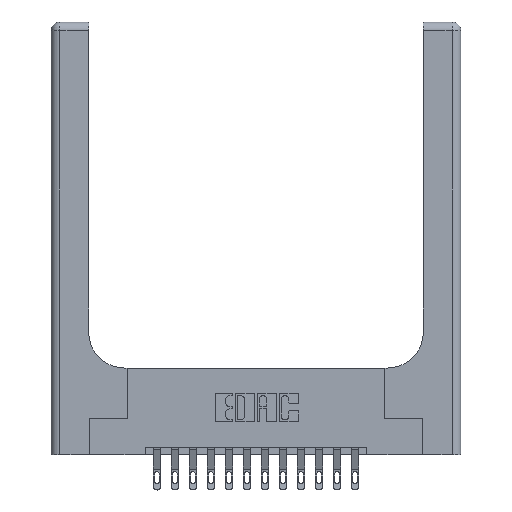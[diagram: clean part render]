
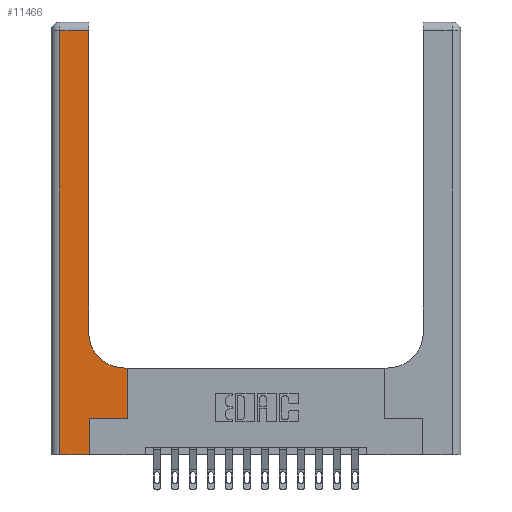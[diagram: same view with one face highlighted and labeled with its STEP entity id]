
A CAD part, top view. The second image highlights one B-rep face of the part: STEP entity #11466.
In plain terms, the highlighted planar face has unit normal (0, 0, 1).
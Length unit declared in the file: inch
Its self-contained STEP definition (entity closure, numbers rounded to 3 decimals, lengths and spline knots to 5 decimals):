
#94 = ORIENTED_EDGE ( 'NONE', *, *, #3642, .T. ) ;
#143 = LINE ( 'NONE', #15207, #8769 ) ;
#165 = DIRECTION ( 'NONE',  ( 1., 0., 0. ) ) ;
#174 = CARTESIAN_POINT ( 'NONE',  ( 0.528, 0.25, 0.37 ) ) ;
#233 = VERTEX_POINT ( 'NONE', #11527 ) ;
#360 = LINE ( 'NONE', #11920, #13364 ) ;
#426 = DIRECTION ( 'NONE',  ( 1., 0., 0. ) ) ;
#514 = ORIENTED_EDGE ( 'NONE', *, *, #17327, .T. ) ;
#552 = VERTEX_POINT ( 'NONE', #10288 ) ;
#580 = CARTESIAN_POINT ( 'NONE',  ( 0.26, 0.6, 0.37 ) ) ;
#708 = CARTESIAN_POINT ( 'NONE',  ( 0., 2.94, 0.37 ) ) ;
#835 = FACE_OUTER_BOUND ( 'NONE', #13564, .T. ) ;
#1359 = LINE ( 'NONE', #708, #5993 ) ;
#1466 = VECTOR ( 'NONE', #4013, 39.37008 ) ;
#1660 = ORIENTED_EDGE ( 'NONE', *, *, #7107, .T. ) ;
#1737 = CARTESIAN_POINT ( 'NONE',  ( 0.26, 2.94, 0.37 ) ) ;
#2424 = VECTOR ( 'NONE', #3629, 39.37008 ) ;
#2548 = CARTESIAN_POINT ( 'NONE',  ( 0.26, 3., 0.37 ) ) ;
#2973 = ORIENTED_EDGE ( 'NONE', *, *, #4875, .T. ) ;
#3167 = CIRCLE ( 'NONE', #9197, 0.25 ) ;
#3177 = VERTEX_POINT ( 'NONE', #11446 ) ;
#3629 = DIRECTION ( 'NONE',  ( 0., 1., 0. ) ) ;
#3642 = EDGE_CURVE ( 'NONE', #552, #5473, #13280, .T. ) ;
#3798 = CARTESIAN_POINT ( 'NONE',  ( 0.265, 0.25, 0.37 ) ) ;
#4013 = DIRECTION ( 'NONE',  ( 0., 1., 0. ) ) ;
#4292 = ORIENTED_EDGE ( 'NONE', *, *, #11459, .T. ) ;
#4373 = CARTESIAN_POINT ( 'NONE',  ( 0.51, 0.6, 0.37 ) ) ;
#4397 = LINE ( 'NONE', #174, #1466 ) ;
#4702 = CARTESIAN_POINT ( 'NONE',  ( 0.265, 0., 0.37 ) ) ;
#4829 = LINE ( 'NONE', #14890, #5902 ) ;
#4875 = EDGE_CURVE ( 'NONE', #11547, #8259, #6325, .T. ) ;
#5184 = CARTESIAN_POINT ( 'NONE',  ( 0.51, 0.85, 0.37 ) ) ;
#5473 = VERTEX_POINT ( 'NONE', #1737 ) ;
#5484 = EDGE_CURVE ( 'NONE', #9661, #11547, #4397, .T. ) ;
#5902 = VECTOR ( 'NONE', #165, 39.37008 ) ;
#5993 = VECTOR ( 'NONE', #12241, 39.37008 ) ;
#6325 = LINE ( 'NONE', #580, #16604 ) ;
#6684 = DIRECTION ( 'NONE',  ( 0., 1., 0. ) ) ;
#7104 = VERTEX_POINT ( 'NONE', #14808 ) ;
#7107 = EDGE_CURVE ( 'NONE', #233, #3177, #360, .T. ) ;
#7856 = EDGE_CURVE ( 'NONE', #5473, #233, #1359, .T. ) ;
#8259 = VERTEX_POINT ( 'NONE', #4373 ) ;
#8502 = DIRECTION ( 'NONE',  ( -1., 0., 0. ) ) ;
#8560 = PLANE ( 'NONE',  #13041 ) ;
#8769 = VECTOR ( 'NONE', #426, 39.37008 ) ;
#9029 = CARTESIAN_POINT ( 'NONE',  ( 0.528, 0.25, 0.37 ) ) ;
#9173 = VERTEX_POINT ( 'NONE', #3798 ) ;
#9197 = AXIS2_PLACEMENT_3D ( 'NONE', #5184, #10015, #12550 ) ;
#9594 = ORIENTED_EDGE ( 'NONE', *, *, #13804, .T. ) ;
#9661 = VERTEX_POINT ( 'NONE', #9029 ) ;
#9811 = DIRECTION ( 'NONE',  ( 0., -1., 0. ) ) ;
#10015 = DIRECTION ( 'NONE',  ( 0., 0., -1. ) ) ;
#10288 = CARTESIAN_POINT ( 'NONE',  ( 0.26, 0.85, 0.37 ) ) ;
#10405 = LINE ( 'NONE', #4702, #2424 ) ;
#11446 = CARTESIAN_POINT ( 'NONE',  ( 0.06, 0., 0.37 ) ) ;
#11459 = EDGE_CURVE ( 'NONE', #3177, #7104, #4829, .T. ) ;
#11466 = ADVANCED_FACE ( 'NONE', ( #835 ), #8560, .F. ) ;
#11527 = CARTESIAN_POINT ( 'NONE',  ( 0.06, 2.94, 0.37 ) ) ;
#11547 = VERTEX_POINT ( 'NONE', #14165 ) ;
#11920 = CARTESIAN_POINT ( 'NONE',  ( 0.06, 3., 0.37 ) ) ;
#12241 = DIRECTION ( 'NONE',  ( -1., 0., 0. ) ) ;
#12550 = DIRECTION ( 'NONE',  ( 1., 0., 0. ) ) ;
#12563 = ORIENTED_EDGE ( 'NONE', *, *, #13828, .T. ) ;
#13041 = AXIS2_PLACEMENT_3D ( 'NONE', #16624, #13859, #8502 ) ;
#13280 = LINE ( 'NONE', #2548, #14562 ) ;
#13364 = VECTOR ( 'NONE', #9811, 39.37008 ) ;
#13564 = EDGE_LOOP ( 'NONE', ( #94, #14661, #1660, #4292, #12563, #9594, #14715, #2973, #514 ) ) ;
#13804 = EDGE_CURVE ( 'NONE', #9173, #9661, #143, .T. ) ;
#13828 = EDGE_CURVE ( 'NONE', #7104, #9173, #10405, .T. ) ;
#13859 = DIRECTION ( 'NONE',  ( 0., 0., -1. ) ) ;
#14165 = CARTESIAN_POINT ( 'NONE',  ( 0.528, 0.6, 0.37 ) ) ;
#14562 = VECTOR ( 'NONE', #6684, 39.37008 ) ;
#14661 = ORIENTED_EDGE ( 'NONE', *, *, #7856, .T. ) ;
#14715 = ORIENTED_EDGE ( 'NONE', *, *, #5484, .T. ) ;
#14808 = CARTESIAN_POINT ( 'NONE',  ( 0.265, 0., 0.37 ) ) ;
#14890 = CARTESIAN_POINT ( 'NONE',  ( 0., 0., 0.37 ) ) ;
#15207 = CARTESIAN_POINT ( 'NONE',  ( 0.265, 0.25, 0.37 ) ) ;
#15299 = DIRECTION ( 'NONE',  ( -1., 0., 0. ) ) ;
#16604 = VECTOR ( 'NONE', #15299, 39.37008 ) ;
#16624 = CARTESIAN_POINT ( 'NONE',  ( 0., 3., 0.37 ) ) ;
#17327 = EDGE_CURVE ( 'NONE', #8259, #552, #3167, .T. ) ;
